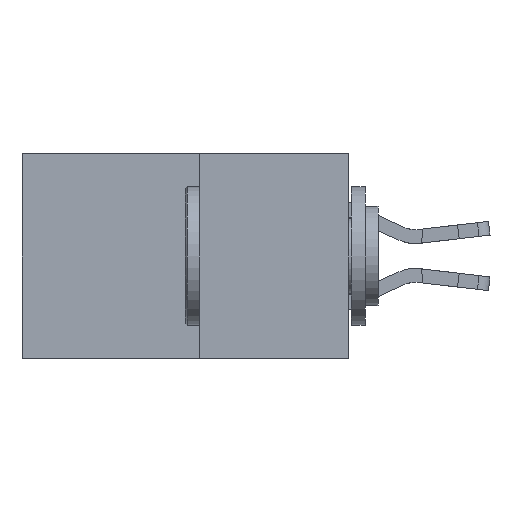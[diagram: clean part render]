
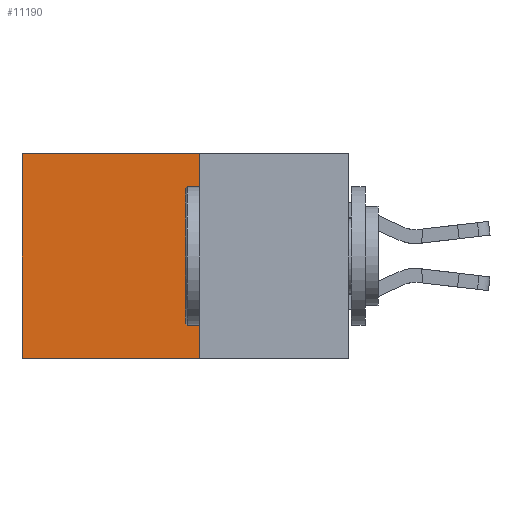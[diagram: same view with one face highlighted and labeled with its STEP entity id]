
A CAD part, left-side view. The second image highlights one B-rep face of the part: STEP entity #11190.
In plain terms, the highlighted planar face has unit normal (-1, 0, 0).
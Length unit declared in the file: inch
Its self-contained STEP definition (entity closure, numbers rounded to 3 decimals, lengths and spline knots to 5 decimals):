
#1 = DIRECTION ( 'NONE',  ( 0., 1., 0. ) ) ;
#767 = LINE ( 'NONE', #18464, #13272 ) ;
#999 = FACE_OUTER_BOUND ( 'NONE', #5981, .T. ) ;
#1085 = CARTESIAN_POINT ( 'NONE',  ( 0.277, 0.59, -0.37 ) ) ;
#1107 = LINE ( 'NONE', #5833, #9620 ) ;
#1877 = EDGE_CURVE ( 'NONE', #10220, #3583, #17181, .T. ) ;
#2168 = DIRECTION ( 'NONE',  ( 0., 0., -1. ) ) ;
#2255 = VECTOR ( 'NONE', #2168, 39.37008 ) ;
#2308 = CARTESIAN_POINT ( 'NONE',  ( 0.277, 0.27, 0. ) ) ;
#2692 = PLANE ( 'NONE',  #14700 ) ;
#3583 = VERTEX_POINT ( 'NONE', #19335 ) ;
#4401 = DIRECTION ( 'NONE',  ( 1., 0., 0. ) ) ;
#5653 = DIRECTION ( 'NONE',  ( 0., 0., -1. ) ) ;
#5833 = CARTESIAN_POINT ( 'NONE',  ( 0.277, 0.59, -0.37 ) ) ;
#5981 = EDGE_LOOP ( 'NONE', ( #8826, #11328, #7228, #6824 ) ) ;
#6520 = EDGE_CURVE ( 'NONE', #3583, #14161, #1107, .T. ) ;
#6824 = ORIENTED_EDGE ( 'NONE', *, *, #1877, .T. ) ;
#7228 = ORIENTED_EDGE ( 'NONE', *, *, #12956, .F. ) ;
#8826 = ORIENTED_EDGE ( 'NONE', *, *, #6520, .T. ) ;
#9374 = CARTESIAN_POINT ( 'NONE',  ( 0.277, 0.27, -0.37 ) ) ;
#9620 = VECTOR ( 'NONE', #5653, 39.37008 ) ;
#10066 = EDGE_CURVE ( 'NONE', #21631, #14161, #767, .T. ) ;
#10220 = VERTEX_POINT ( 'NONE', #10555 ) ;
#10555 = CARTESIAN_POINT ( 'NONE',  ( 0.277, 0.27, 0. ) ) ;
#10674 = CARTESIAN_POINT ( 'NONE',  ( 0.277, 0.27, -0.37 ) ) ;
#11190 = ADVANCED_FACE ( 'NONE', ( #999 ), #2692, .F. ) ;
#11328 = ORIENTED_EDGE ( 'NONE', *, *, #10066, .F. ) ;
#11844 = DIRECTION ( 'NONE',  ( 0., 1., 0. ) ) ;
#12956 = EDGE_CURVE ( 'NONE', #10220, #21631, #20163, .T. ) ;
#13272 = VECTOR ( 'NONE', #11844, 39.37008 ) ;
#14161 = VERTEX_POINT ( 'NONE', #1085 ) ;
#14586 = CARTESIAN_POINT ( 'NONE',  ( 0.277, 0.27, -0.37 ) ) ;
#14700 = AXIS2_PLACEMENT_3D ( 'NONE', #14586, #4401, #16294 ) ;
#16157 = VECTOR ( 'NONE', #1, 39.37008 ) ;
#16294 = DIRECTION ( 'NONE',  ( 0., 0., -1. ) ) ;
#17181 = LINE ( 'NONE', #2308, #16157 ) ;
#18464 = CARTESIAN_POINT ( 'NONE',  ( 0.277, 0.27, -0.37 ) ) ;
#19335 = CARTESIAN_POINT ( 'NONE',  ( 0.277, 0.59, 0. ) ) ;
#20163 = LINE ( 'NONE', #10674, #2255 ) ;
#21631 = VERTEX_POINT ( 'NONE', #9374 ) ;
